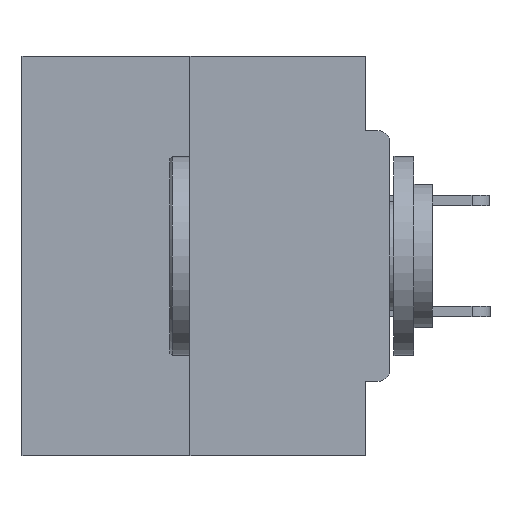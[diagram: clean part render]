
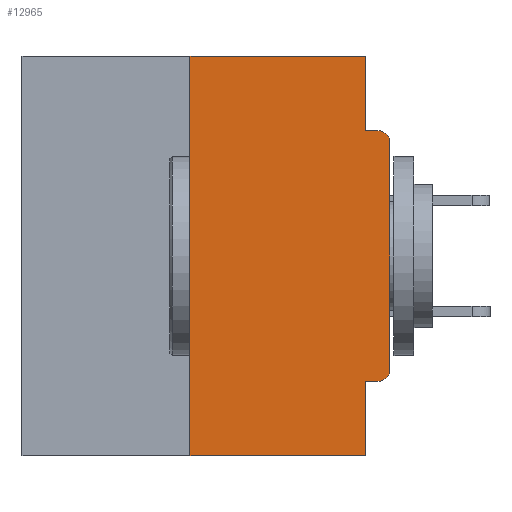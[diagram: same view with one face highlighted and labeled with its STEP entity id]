
A CAD part, left-side view. The second image highlights one B-rep face of the part: STEP entity #12965.
In plain terms, the highlighted planar face has unit normal (-1, 0, 0).
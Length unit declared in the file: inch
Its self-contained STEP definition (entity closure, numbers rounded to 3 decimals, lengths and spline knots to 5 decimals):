
#111 = ORIENTED_EDGE ( 'NONE', *, *, #27492, .T. ) ;
#1632 = DIRECTION ( 'NONE',  ( 0., 0., 1. ) ) ;
#1826 = FACE_OUTER_BOUND ( 'NONE', #1948, .T. ) ;
#1948 = EDGE_LOOP ( 'NONE', ( #2550, #3977, #11857, #27406, #7022, #13762, #111, #15086, #15816, #6840 ) ) ;
#2550 = ORIENTED_EDGE ( 'NONE', *, *, #5949, .F. ) ;
#2599 = CARTESIAN_POINT ( 'NONE',  ( 0., 0.46, -0.5 ) ) ;
#2789 = AXIS2_PLACEMENT_3D ( 'NONE', #19323, #3177, #5869 ) ;
#3177 = DIRECTION ( 'NONE',  ( -1., 0., 0. ) ) ;
#3484 = EDGE_CURVE ( 'NONE', #34215, #4025, #14573, .T. ) ;
#3733 = DIRECTION ( 'NONE',  ( 0., -1., 0. ) ) ;
#3937 = CARTESIAN_POINT ( 'NONE',  ( 0., 0.031, -0.5 ) ) ;
#3977 = ORIENTED_EDGE ( 'NONE', *, *, #6711, .F. ) ;
#4025 = VERTEX_POINT ( 'NONE', #26448 ) ;
#4033 = VERTEX_POINT ( 'NONE', #34430 ) ;
#4297 = DIRECTION ( 'NONE',  ( -1., 0., 0. ) ) ;
#4410 = VECTOR ( 'NONE', #23928, 39.37008 ) ;
#4475 = VECTOR ( 'NONE', #33361, 39.37008 ) ;
#4513 = VECTOR ( 'NONE', #21608, 39.37008 ) ;
#5402 = DIRECTION ( 'NONE',  ( 0., 1., 0. ) ) ;
#5456 = VERTEX_POINT ( 'NONE', #34353 ) ;
#5869 = DIRECTION ( 'NONE',  ( 0., 0., -1. ) ) ;
#5949 = EDGE_CURVE ( 'NONE', #5456, #4033, #24382, .T. ) ;
#6711 = EDGE_CURVE ( 'NONE', #11156, #5456, #9618, .T. ) ;
#6840 = ORIENTED_EDGE ( 'NONE', *, *, #33694, .F. ) ;
#7022 = ORIENTED_EDGE ( 'NONE', *, *, #34141, .F. ) ;
#8105 = CARTESIAN_POINT ( 'NONE',  ( 0., 0.015, -0.4065 ) ) ;
#8912 = AXIS2_PLACEMENT_3D ( 'NONE', #18196, #31957, #26456 ) ;
#9301 = VERTEX_POINT ( 'NONE', #32004 ) ;
#9618 = LINE ( 'NONE', #28941, #14291 ) ;
#10042 = VECTOR ( 'NONE', #3733, 39.37008 ) ;
#11043 = CARTESIAN_POINT ( 'NONE',  ( 0., 0.031, -0.0935 ) ) ;
#11156 = VERTEX_POINT ( 'NONE', #20575 ) ;
#11270 = VERTEX_POINT ( 'NONE', #27152 ) ;
#11631 = LINE ( 'NONE', #3937, #4475 ) ;
#11676 = LINE ( 'NONE', #34761, #4513 ) ;
#11857 = ORIENTED_EDGE ( 'NONE', *, *, #18043, .T. ) ;
#12034 = DIRECTION ( 'NONE',  ( 0., 0., -1. ) ) ;
#12092 = CARTESIAN_POINT ( 'NONE',  ( 0., 0.46, 0. ) ) ;
#12965 = ADVANCED_FACE ( 'NONE', ( #1826 ), #34200, .F. ) ;
#13762 = ORIENTED_EDGE ( 'NONE', *, *, #31791, .T. ) ;
#14291 = VECTOR ( 'NONE', #1632, 39.37008 ) ;
#14573 = LINE ( 'NONE', #29413, #17095 ) ;
#14694 = VERTEX_POINT ( 'NONE', #21724 ) ;
#15086 = ORIENTED_EDGE ( 'NONE', *, *, #30660, .T. ) ;
#15816 = ORIENTED_EDGE ( 'NONE', *, *, #3484, .F. ) ;
#16247 = CARTESIAN_POINT ( 'NONE',  ( 0., 0., -0.4065 ) ) ;
#16646 = EDGE_CURVE ( 'NONE', #14694, #9301, #11631, .T. ) ;
#17095 = VECTOR ( 'NONE', #19166, 39.37008 ) ;
#17720 = DIRECTION ( 'NONE',  ( 0., 0., -1. ) ) ;
#18043 = EDGE_CURVE ( 'NONE', #11156, #9301, #22152, .T. ) ;
#18196 = CARTESIAN_POINT ( 'NONE',  ( 0., 0.46, 0. ) ) ;
#19166 = DIRECTION ( 'NONE',  ( 0., -1., 0. ) ) ;
#19323 = CARTESIAN_POINT ( 'NONE',  ( 0., 0.015, -0.3915 ) ) ;
#20405 = CARTESIAN_POINT ( 'NONE',  ( 0., 0.031, 0. ) ) ;
#20571 = CARTESIAN_POINT ( 'NONE',  ( 0., 0.015, -0.1085 ) ) ;
#20575 = CARTESIAN_POINT ( 'NONE',  ( 0., 0.25, -0.5 ) ) ;
#21363 = CIRCLE ( 'NONE', #2789, 0.015 ) ;
#21608 = DIRECTION ( 'NONE',  ( 0., 0., 1. ) ) ;
#21724 = CARTESIAN_POINT ( 'NONE',  ( 0., 0.031, -0.4065 ) ) ;
#22077 = VECTOR ( 'NONE', #5402, 39.37008 ) ;
#22152 = LINE ( 'NONE', #2599, #4410 ) ;
#22676 = VERTEX_POINT ( 'NONE', #25813 ) ;
#23272 = LINE ( 'NONE', #16247, #22077 ) ;
#23928 = DIRECTION ( 'NONE',  ( 0., -1., 0. ) ) ;
#24382 = LINE ( 'NONE', #12092, #10042 ) ;
#25813 = CARTESIAN_POINT ( 'NONE',  ( 0., 0., -0.3915 ) ) ;
#26448 = CARTESIAN_POINT ( 'NONE',  ( 0., 0.015, -0.0935 ) ) ;
#26456 = DIRECTION ( 'NONE',  ( 0., 0., -1. ) ) ;
#27152 = CARTESIAN_POINT ( 'NONE',  ( 0., 0., -0.1085 ) ) ;
#27406 = ORIENTED_EDGE ( 'NONE', *, *, #16646, .F. ) ;
#27492 = EDGE_CURVE ( 'NONE', #22676, #11270, #11676, .T. ) ;
#28732 = CIRCLE ( 'NONE', #30519, 0.015 ) ;
#28941 = CARTESIAN_POINT ( 'NONE',  ( 0., 0.25, 0. ) ) ;
#29413 = CARTESIAN_POINT ( 'NONE',  ( 0., 0., -0.0935 ) ) ;
#29765 = VERTEX_POINT ( 'NONE', #8105 ) ;
#30519 = AXIS2_PLACEMENT_3D ( 'NONE', #20571, #4297, #17720 ) ;
#30660 = EDGE_CURVE ( 'NONE', #11270, #4025, #28732, .T. ) ;
#31791 = EDGE_CURVE ( 'NONE', #29765, #22676, #21363, .T. ) ;
#31957 = DIRECTION ( 'NONE',  ( 1., 0., 0. ) ) ;
#32004 = CARTESIAN_POINT ( 'NONE',  ( 0., 0.031, -0.5 ) ) ;
#32561 = VECTOR ( 'NONE', #12034, 39.37008 ) ;
#33361 = DIRECTION ( 'NONE',  ( 0., 0., -1. ) ) ;
#33694 = EDGE_CURVE ( 'NONE', #4033, #34215, #34666, .T. ) ;
#34141 = EDGE_CURVE ( 'NONE', #29765, #14694, #23272, .T. ) ;
#34200 = PLANE ( 'NONE',  #8912 ) ;
#34215 = VERTEX_POINT ( 'NONE', #11043 ) ;
#34353 = CARTESIAN_POINT ( 'NONE',  ( 0., 0.25, 0. ) ) ;
#34430 = CARTESIAN_POINT ( 'NONE',  ( 0., 0.031, 0. ) ) ;
#34666 = LINE ( 'NONE', #20405, #32561 ) ;
#34761 = CARTESIAN_POINT ( 'NONE',  ( 0., 0., 0. ) ) ;
